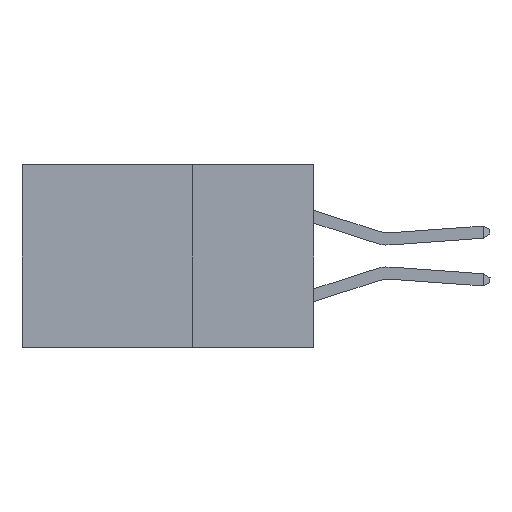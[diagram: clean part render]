
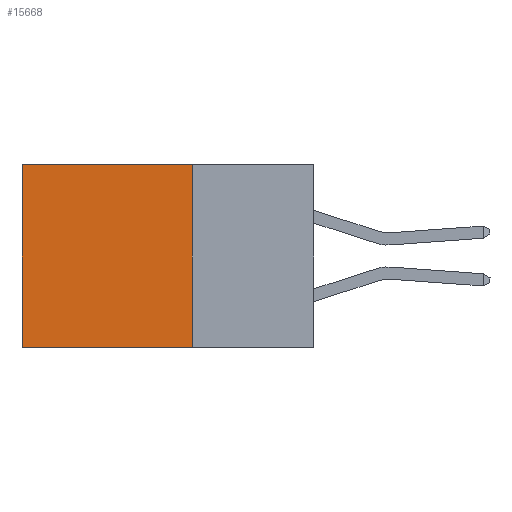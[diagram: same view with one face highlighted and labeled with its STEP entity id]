
A CAD part, left-side view. The second image highlights one B-rep face of the part: STEP entity #15668.
In plain terms, the highlighted planar face has unit normal (-1, 0, 0).
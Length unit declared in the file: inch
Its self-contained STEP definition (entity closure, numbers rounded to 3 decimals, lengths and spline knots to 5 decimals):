
#93 = VECTOR ( 'NONE', #12275, 39.37008 ) ;
#184 = LINE ( 'NONE', #1571, #13121 ) ;
#394 = FACE_OUTER_BOUND ( 'NONE', #16707, .T. ) ;
#581 = LINE ( 'NONE', #4255, #9621 ) ;
#1224 = ORIENTED_EDGE ( 'NONE', *, *, #19075, .T. ) ;
#1571 = CARTESIAN_POINT ( 'NONE',  ( 0.2875, 0.25, -0.375 ) ) ;
#1884 = VERTEX_POINT ( 'NONE', #12738 ) ;
#3059 = ORIENTED_EDGE ( 'NONE', *, *, #6414, .F. ) ;
#3277 = CARTESIAN_POINT ( 'NONE',  ( 0.2875, 0.25, 0. ) ) ;
#3684 = EDGE_CURVE ( 'NONE', #14899, #1884, #184, .T. ) ;
#3845 = VERTEX_POINT ( 'NONE', #13982 ) ;
#4255 = CARTESIAN_POINT ( 'NONE',  ( 0.2875, 0.25, -0.375 ) ) ;
#6414 = EDGE_CURVE ( 'NONE', #11717, #14899, #581, .T. ) ;
#8410 = VECTOR ( 'NONE', #14151, 39.37008 ) ;
#9621 = VECTOR ( 'NONE', #13725, 39.37008 ) ;
#10074 = CARTESIAN_POINT ( 'NONE',  ( 0.2875, 0.25, -0.375 ) ) ;
#10581 = CARTESIAN_POINT ( 'NONE',  ( 0.2875, 0.6, -0.375 ) ) ;
#11717 = VERTEX_POINT ( 'NONE', #12546 ) ;
#11905 = DIRECTION ( 'NONE',  ( 0., 0., -1. ) ) ;
#12153 = ORIENTED_EDGE ( 'NONE', *, *, #17315, .T. ) ;
#12275 = DIRECTION ( 'NONE',  ( 0., 0., -1. ) ) ;
#12546 = CARTESIAN_POINT ( 'NONE',  ( 0.2875, 0.25, 0. ) ) ;
#12738 = CARTESIAN_POINT ( 'NONE',  ( 0.2875, 0.6, -0.375 ) ) ;
#12832 = LINE ( 'NONE', #3277, #8410 ) ;
#13121 = VECTOR ( 'NONE', #15525, 39.37008 ) ;
#13725 = DIRECTION ( 'NONE',  ( 0., 0., -1. ) ) ;
#13878 = ORIENTED_EDGE ( 'NONE', *, *, #3684, .F. ) ;
#13982 = CARTESIAN_POINT ( 'NONE',  ( 0.2875, 0.6, 0. ) ) ;
#13986 = LINE ( 'NONE', #10581, #93 ) ;
#14151 = DIRECTION ( 'NONE',  ( 0., 1., 0. ) ) ;
#14539 = PLANE ( 'NONE',  #15733 ) ;
#14899 = VERTEX_POINT ( 'NONE', #10074 ) ;
#15525 = DIRECTION ( 'NONE',  ( 0., 1., 0. ) ) ;
#15668 = ADVANCED_FACE ( 'NONE', ( #394 ), #14539, .F. ) ;
#15733 = AXIS2_PLACEMENT_3D ( 'NONE', #16531, #18052, #11905 ) ;
#16531 = CARTESIAN_POINT ( 'NONE',  ( 0.2875, 0.25, -0.375 ) ) ;
#16707 = EDGE_LOOP ( 'NONE', ( #1224, #13878, #3059, #12153 ) ) ;
#17315 = EDGE_CURVE ( 'NONE', #11717, #3845, #12832, .T. ) ;
#18052 = DIRECTION ( 'NONE',  ( 1., 0., 0. ) ) ;
#19075 = EDGE_CURVE ( 'NONE', #3845, #1884, #13986, .T. ) ;
